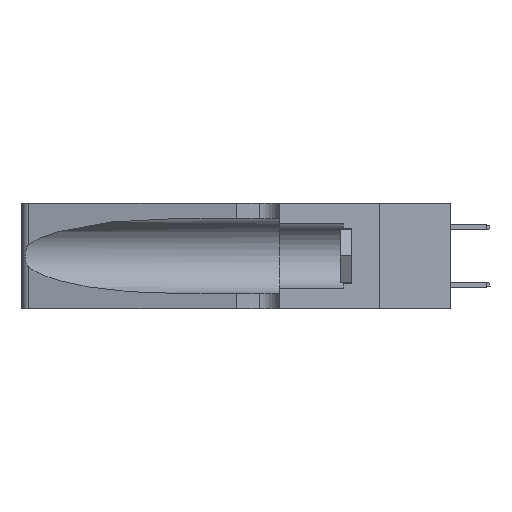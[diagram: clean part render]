
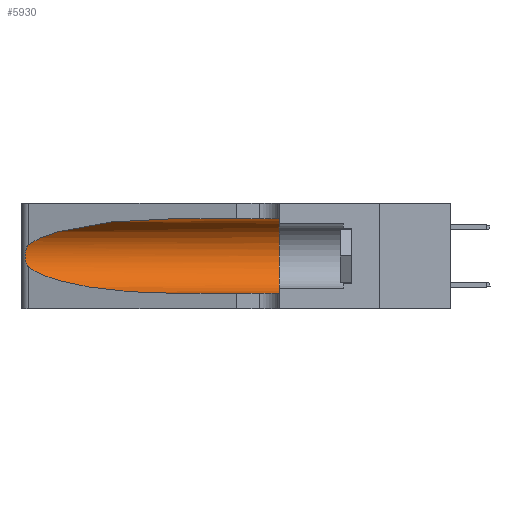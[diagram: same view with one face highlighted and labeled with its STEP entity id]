
A CAD part, left-side view. The second image highlights one B-rep face of the part: STEP entity #5930.
In plain terms, the highlighted cylindrical face has radius 3.308 mm (diameter 6.617 mm), a partial arc.
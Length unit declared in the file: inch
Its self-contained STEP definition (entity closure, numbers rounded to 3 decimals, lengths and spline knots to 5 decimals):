
#67 = DIRECTION ( 'NONE',  ( 0., 1., 0. ) ) ;
#128 = EDGE_CURVE ( 'NONE', #14551, #11078, #4714, .T. ) ;
#264 = LINE ( 'NONE', #9905, #11759 ) ;
#569 = CARTESIAN_POINT ( 'NONE',  ( 0.26075, 1.23896, 0.178 ) ) ;
#672 = DIRECTION ( 'NONE',  ( 0., -1., 0. ) ) ;
#786 = CARTESIAN_POINT ( 'NONE',  ( 0.25487, 1.22718, 0.22369 ) ) ;
#976 = CARTESIAN_POINT ( 'NONE',  ( 0.25854, 1.2359, 0.20912 ) ) ;
#1347 = CARTESIAN_POINT ( 'NONE',  ( 0.25555, 1.22993, 0.14849 ) ) ;
#1734 = CARTESIAN_POINT ( 'NONE',  ( 0.1305, 0.72297, 0.05475 ) ) ;
#2217 = CARTESIAN_POINT ( 'NONE',  ( 0.25555, 1.22994, 0.2215 ) ) ;
#3171 = CARTESIAN_POINT ( 'NONE',  ( 0.18966, 0.96281, 0.05475 ) ) ;
#3474 = ORIENTED_EDGE ( 'NONE', *, *, #128, .F. ) ;
#3798 = CARTESIAN_POINT ( 'NONE',  ( 0.1305, 1.61858, 0.185 ) ) ;
#3838 = ORIENTED_EDGE ( 'NONE', *, *, #4442, .T. ) ;
#3883 = CYLINDRICAL_SURFACE ( 'NONE', #5637, 0.13025 ) ;
#4442 = EDGE_CURVE ( 'NONE', #12238, #6437, #5734, .T. ) ;
#4714 = CIRCLE ( 'NONE', #14673, 0.13025 ) ;
#5450 = CARTESIAN_POINT ( 'NONE',  ( 0.25487, 1.22718, 0.14631 ) ) ;
#5637 = AXIS2_PLACEMENT_3D ( 'NONE', #3798, #6265, #9041 ) ;
#5734 = B_SPLINE_CURVE_WITH_KNOTS ( 'NONE', 3,
 ( #786, #2217, #6306, #13187, #976, #8608, #12790, #569, #12445, #11100, #16552, #11907, #1347, #5450 ),
 .UNSPECIFIED., .F., .F.,
 ( 4, 2, 2, 2, 2, 2, 4 ),
 ( 0., 0.00027, 0.00053, 0.00107, 0.0016, 0.00187, 0.00214 ),
 .UNSPECIFIED. ) ;
#5930 = ADVANCED_FACE ( 'NONE', ( #10464 ), #3883, .F. ) ;
#6265 = DIRECTION ( 'NONE',  ( 0., -1., 0. ) ) ;
#6306 = CARTESIAN_POINT ( 'NONE',  ( 0.25639, 1.23184, 0.21858 ) ) ;
#6437 = VERTEX_POINT ( 'NONE', #13819 ) ;
#6904 = CARTESIAN_POINT ( 'NONE',  ( 0.1305, 0.35, 0.31525 ) ) ;
#7297 = VECTOR ( 'NONE', #672, 39.37008 ) ;
#7922 = LINE ( 'NONE', #17437, #7297 ) ;
#7974 = CARTESIAN_POINT ( 'NONE',  ( 0.25487, 1.22718, 0.22369 ) ) ;
#8608 = CARTESIAN_POINT ( 'NONE',  ( 0.26018, 1.23835, 0.19895 ) ) ;
#8839 = CARTESIAN_POINT ( 'NONE',  ( 0.2373, 1.15595, 0.08982 ) ) ;
#8937 =( BOUNDED_CURVE ( )  B_SPLINE_CURVE ( 3, ( #15618, #8839, #3171, #1734 ),
 .UNSPECIFIED., .F., .F. ) 
 B_SPLINE_CURVE_WITH_KNOTS ( ( 4, 4 ),
 ( 3.44316, 4.71239 ),
 .UNSPECIFIED. ) 
 CURVE ( )  GEOMETRIC_REPRESENTATION_ITEM ( )  RATIONAL_B_SPLINE_CURVE ( ( 1., 0.87, 0.87, 1. ) ) 
 REPRESENTATION_ITEM ( '' )  );
#9041 = DIRECTION ( 'NONE',  ( 0., 0., -1. ) ) ;
#9168 = CARTESIAN_POINT ( 'NONE',  ( 0.18966, 0.96281, 0.31525 ) ) ;
#9407 = ORIENTED_EDGE ( 'NONE', *, *, #16983, .T. ) ;
#9782 = CARTESIAN_POINT ( 'NONE',  ( 0.1305, 0.72297, 0.05475 ) ) ;
#9785 = EDGE_CURVE ( 'NONE', #6437, #12805, #8937, .T. ) ;
#9905 = CARTESIAN_POINT ( 'NONE',  ( 0.1305, 1.61858, 0.05475 ) ) ;
#10464 = FACE_OUTER_BOUND ( 'NONE', #16804, .T. ) ;
#10494 = CARTESIAN_POINT ( 'NONE',  ( 0.1305, 0.72297, 0.31525 ) ) ;
#10679 = CARTESIAN_POINT ( 'NONE',  ( 0.2373, 1.15595, 0.28018 ) ) ;
#11078 = VERTEX_POINT ( 'NONE', #12538 ) ;
#11100 = CARTESIAN_POINT ( 'NONE',  ( 0.25856, 1.23593, 0.16098 ) ) ;
#11162 = EDGE_CURVE ( 'NONE', #15543, #14551, #7922, .T. ) ;
#11759 = VECTOR ( 'NONE', #12566, 39.37008 ) ;
#11907 = CARTESIAN_POINT ( 'NONE',  ( 0.25639, 1.23186, 0.15144 ) ) ;
#12238 = VERTEX_POINT ( 'NONE', #14758 ) ;
#12445 = CARTESIAN_POINT ( 'NONE',  ( 0.26017, 1.23833, 0.17102 ) ) ;
#12538 = CARTESIAN_POINT ( 'NONE',  ( 0.1305, 0.35, 0.05475 ) ) ;
#12566 = DIRECTION ( 'NONE',  ( 0., -1., 0. ) ) ;
#12790 = CARTESIAN_POINT ( 'NONE',  ( 0.26075, 1.23896, 0.19203 ) ) ;
#12805 = VERTEX_POINT ( 'NONE', #9782 ) ;
#13028 = EDGE_CURVE ( 'NONE', #15543, #12238, #17395, .T. ) ;
#13187 = CARTESIAN_POINT ( 'NONE',  ( 0.25787, 1.23484, 0.2124 ) ) ;
#13819 = CARTESIAN_POINT ( 'NONE',  ( 0.25487, 1.22718, 0.14631 ) ) ;
#14225 = CARTESIAN_POINT ( 'NONE',  ( 0.1305, 0.72297, 0.31525 ) ) ;
#14551 = VERTEX_POINT ( 'NONE', #6904 ) ;
#14673 = AXIS2_PLACEMENT_3D ( 'NONE', #15137, #67, #15044 ) ;
#14758 = CARTESIAN_POINT ( 'NONE',  ( 0.25487, 1.22718, 0.22369 ) ) ;
#15044 = DIRECTION ( 'NONE',  ( 0., 0., 1. ) ) ;
#15137 = CARTESIAN_POINT ( 'NONE',  ( 0.1305, 0.35, 0.185 ) ) ;
#15543 = VERTEX_POINT ( 'NONE', #14225 ) ;
#15618 = CARTESIAN_POINT ( 'NONE',  ( 0.25487, 1.22718, 0.14631 ) ) ;
#15631 = ORIENTED_EDGE ( 'NONE', *, *, #11162, .F. ) ;
#15865 = ORIENTED_EDGE ( 'NONE', *, *, #9785, .T. ) ;
#16552 = CARTESIAN_POINT ( 'NONE',  ( 0.25789, 1.23486, 0.15765 ) ) ;
#16804 = EDGE_LOOP ( 'NONE', ( #16996, #3838, #15865, #9407, #3474, #15631 ) ) ;
#16983 = EDGE_CURVE ( 'NONE', #12805, #11078, #264, .T. ) ;
#16996 = ORIENTED_EDGE ( 'NONE', *, *, #13028, .T. ) ;
#17395 =( BOUNDED_CURVE ( )  B_SPLINE_CURVE ( 3, ( #10494, #9168, #10679, #7974 ),
 .UNSPECIFIED., .F., .F. ) 
 B_SPLINE_CURVE_WITH_KNOTS ( ( 4, 4 ),
 ( 1.5708, 2.84003 ),
 .UNSPECIFIED. ) 
 CURVE ( )  GEOMETRIC_REPRESENTATION_ITEM ( )  RATIONAL_B_SPLINE_CURVE ( ( 1., 0.87, 0.87, 1. ) ) 
 REPRESENTATION_ITEM ( '' )  );
#17437 = CARTESIAN_POINT ( 'NONE',  ( 0.1305, 1.61858, 0.31525 ) ) ;
